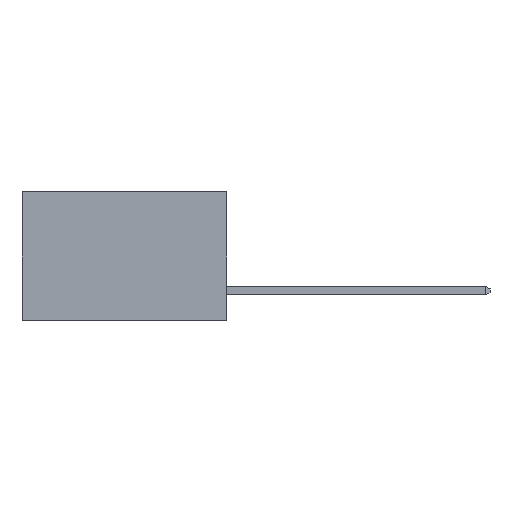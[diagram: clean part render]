
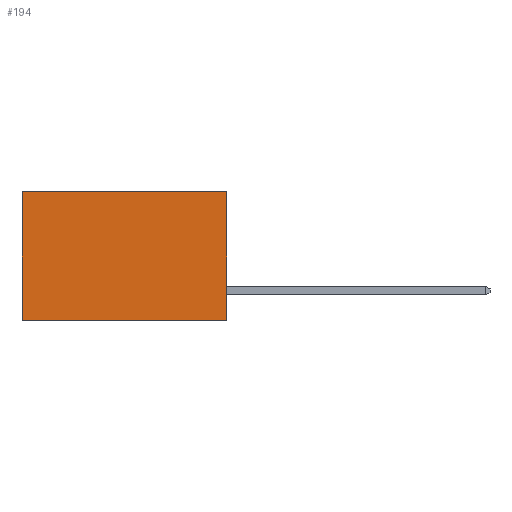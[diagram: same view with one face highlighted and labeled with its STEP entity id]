
A CAD part, left-side view. The second image highlights one B-rep face of the part: STEP entity #194.
In plain terms, the highlighted planar face has unit normal (-1, 0, 0).
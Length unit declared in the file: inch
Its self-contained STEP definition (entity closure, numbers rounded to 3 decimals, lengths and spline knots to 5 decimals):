
#44 = VECTOR ( 'NONE', #977, 39.37008 ) ;
#194 = ADVANCED_FACE ( 'NONE', ( #4932 ), #5106, .F. ) ;
#258 = ORIENTED_EDGE ( 'NONE', *, *, #6959, .F. ) ;
#315 = ORIENTED_EDGE ( 'NONE', *, *, #1414, .F. ) ;
#357 = VECTOR ( 'NONE', #801, 39.37008 ) ;
#449 = VECTOR ( 'NONE', #1972, 39.37008 ) ;
#623 = CARTESIAN_POINT ( 'NONE',  ( 0.277, 0., 0. ) ) ;
#731 = ORIENTED_EDGE ( 'NONE', *, *, #7447, .T. ) ;
#760 = LINE ( 'NONE', #623, #357 ) ;
#764 = CARTESIAN_POINT ( 'NONE',  ( 0.277, 0., -0.37 ) ) ;
#801 = DIRECTION ( 'NONE',  ( 0., 1., 0. ) ) ;
#861 = EDGE_CURVE ( 'NONE', #6308, #4221, #2158, .T. ) ;
#977 = DIRECTION ( 'NONE',  ( 0., 0., -1. ) ) ;
#1089 = ORIENTED_EDGE ( 'NONE', *, *, #861, .T. ) ;
#1360 = CARTESIAN_POINT ( 'NONE',  ( 0.277, 0.59, -0.37 ) ) ;
#1414 = EDGE_CURVE ( 'NONE', #2345, #4221, #6885, .T. ) ;
#1747 = VECTOR ( 'NONE', #1912, 39.37008 ) ;
#1790 = EDGE_LOOP ( 'NONE', ( #1089, #315, #258, #731 ) ) ;
#1903 = CARTESIAN_POINT ( 'NONE',  ( 0.277, 0., -0.37 ) ) ;
#1912 = DIRECTION ( 'NONE',  ( 0., 1., 0. ) ) ;
#1936 = CARTESIAN_POINT ( 'NONE',  ( 0.277, 0., -0.37 ) ) ;
#1972 = DIRECTION ( 'NONE',  ( 0., 0., -1. ) ) ;
#2158 = LINE ( 'NONE', #1360, #449 ) ;
#2345 = VERTEX_POINT ( 'NONE', #4458 ) ;
#2782 = VERTEX_POINT ( 'NONE', #4767 ) ;
#3446 = CARTESIAN_POINT ( 'NONE',  ( 0.277, 0.59, 0. ) ) ;
#3461 = LINE ( 'NONE', #764, #44 ) ;
#4221 = VERTEX_POINT ( 'NONE', #7527 ) ;
#4345 = DIRECTION ( 'NONE',  ( 0., 0., -1. ) ) ;
#4458 = CARTESIAN_POINT ( 'NONE',  ( 0.277, 0., -0.37 ) ) ;
#4767 = CARTESIAN_POINT ( 'NONE',  ( 0.277, 0., 0. ) ) ;
#4932 = FACE_OUTER_BOUND ( 'NONE', #1790, .T. ) ;
#5106 = PLANE ( 'NONE',  #7880 ) ;
#5715 = DIRECTION ( 'NONE',  ( 1., 0., 0. ) ) ;
#6308 = VERTEX_POINT ( 'NONE', #3446 ) ;
#6885 = LINE ( 'NONE', #1936, #1747 ) ;
#6959 = EDGE_CURVE ( 'NONE', #2782, #2345, #3461, .T. ) ;
#7447 = EDGE_CURVE ( 'NONE', #2782, #6308, #760, .T. ) ;
#7527 = CARTESIAN_POINT ( 'NONE',  ( 0.277, 0.59, -0.37 ) ) ;
#7880 = AXIS2_PLACEMENT_3D ( 'NONE', #1903, #5715, #4345 ) ;
